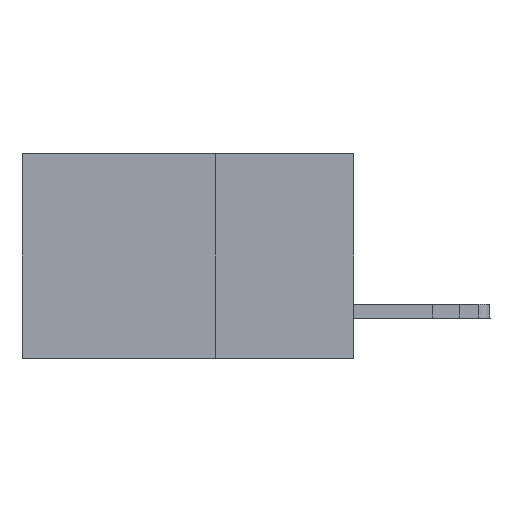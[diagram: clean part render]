
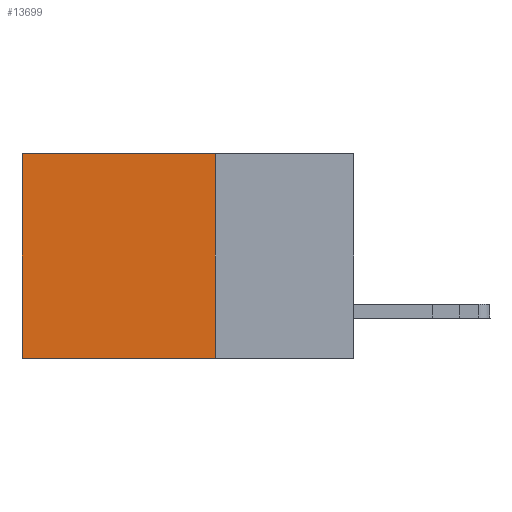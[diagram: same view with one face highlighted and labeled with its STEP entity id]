
A CAD part, left-side view. The second image highlights one B-rep face of the part: STEP entity #13699.
In plain terms, the highlighted planar face has unit normal (-1, 0, 0).
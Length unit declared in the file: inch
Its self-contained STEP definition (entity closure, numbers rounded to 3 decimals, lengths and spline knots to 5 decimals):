
#2628 = EDGE_CURVE ( 'NONE', #17980, #8611, #17893, .T. ) ;
#4429 = CARTESIAN_POINT ( 'NONE',  ( 0.2875, 0.6, -0.37 ) ) ;
#4504 = ORIENTED_EDGE ( 'NONE', *, *, #2628, .F. ) ;
#5147 = VERTEX_POINT ( 'NONE', #19702 ) ;
#5557 = CARTESIAN_POINT ( 'NONE',  ( 0.2875, 0.25, -0.37 ) ) ;
#5573 = LINE ( 'NONE', #12641, #16960 ) ;
#5716 = AXIS2_PLACEMENT_3D ( 'NONE', #15946, #6931, #21286 ) ;
#5737 = DIRECTION ( 'NONE',  ( 0., 1., 0. ) ) ;
#6763 = VECTOR ( 'NONE', #14958, 39.37008 ) ;
#6931 = DIRECTION ( 'NONE',  ( 1., 0., 0. ) ) ;
#8611 = VERTEX_POINT ( 'NONE', #4429 ) ;
#11415 = ORIENTED_EDGE ( 'NONE', *, *, #11770, .F. ) ;
#11636 = VERTEX_POINT ( 'NONE', #18573 ) ;
#11770 = EDGE_CURVE ( 'NONE', #11636, #17980, #13558, .T. ) ;
#12641 = CARTESIAN_POINT ( 'NONE',  ( 0.2875, 0.6, 0. ) ) ;
#13558 = LINE ( 'NONE', #16676, #6763 ) ;
#13699 = ADVANCED_FACE ( 'NONE', ( #19322 ), #15726, .F. ) ;
#13916 = VECTOR ( 'NONE', #5737, 39.37008 ) ;
#14958 = DIRECTION ( 'NONE',  ( 0., 0., -1. ) ) ;
#15478 = EDGE_CURVE ( 'NONE', #11636, #5147, #21607, .T. ) ;
#15726 = PLANE ( 'NONE',  #5716 ) ;
#15946 = CARTESIAN_POINT ( 'NONE',  ( 0.2875, 0.25, 0. ) ) ;
#16388 = CARTESIAN_POINT ( 'NONE',  ( 0.2875, 0.25, 0. ) ) ;
#16486 = ORIENTED_EDGE ( 'NONE', *, *, #15478, .T. ) ;
#16676 = CARTESIAN_POINT ( 'NONE',  ( 0.2875, 0.25, 0. ) ) ;
#16782 = EDGE_LOOP ( 'NONE', ( #22428, #4504, #11415, #16486 ) ) ;
#16960 = VECTOR ( 'NONE', #21561, 39.37008 ) ;
#17401 = VECTOR ( 'NONE', #19511, 39.37008 ) ;
#17767 = CARTESIAN_POINT ( 'NONE',  ( 0.2875, 0.25, -0.37 ) ) ;
#17893 = LINE ( 'NONE', #17767, #17401 ) ;
#17980 = VERTEX_POINT ( 'NONE', #5557 ) ;
#18573 = CARTESIAN_POINT ( 'NONE',  ( 0.2875, 0.25, 0. ) ) ;
#19322 = FACE_OUTER_BOUND ( 'NONE', #16782, .T. ) ;
#19511 = DIRECTION ( 'NONE',  ( 0., 1., 0. ) ) ;
#19702 = CARTESIAN_POINT ( 'NONE',  ( 0.2875, 0.6, 0. ) ) ;
#20019 = EDGE_CURVE ( 'NONE', #5147, #8611, #5573, .T. ) ;
#21286 = DIRECTION ( 'NONE',  ( 0., 0., -1. ) ) ;
#21561 = DIRECTION ( 'NONE',  ( 0., 0., -1. ) ) ;
#21607 = LINE ( 'NONE', #16388, #13916 ) ;
#22428 = ORIENTED_EDGE ( 'NONE', *, *, #20019, .T. ) ;
